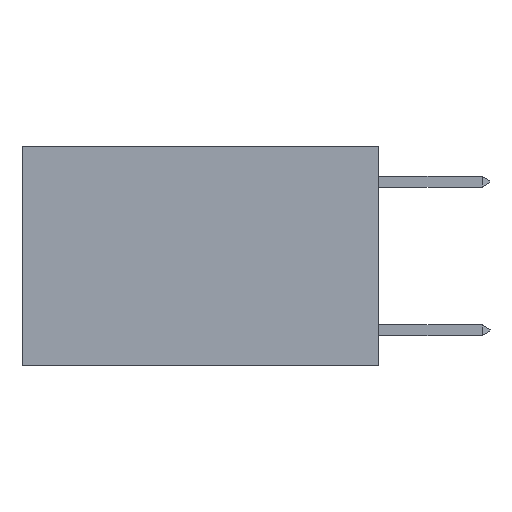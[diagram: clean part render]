
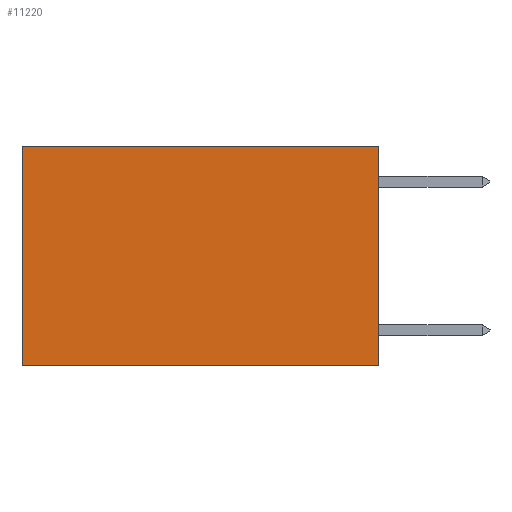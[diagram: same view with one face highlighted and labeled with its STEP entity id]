
A CAD part, left-side view. The second image highlights one B-rep face of the part: STEP entity #11220.
In plain terms, the highlighted planar face has unit normal (-1, 0, 0).
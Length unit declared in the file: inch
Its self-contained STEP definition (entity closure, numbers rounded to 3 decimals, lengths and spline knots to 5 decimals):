
#26 = VERTEX_POINT ( 'NONE', #25064 ) ;
#434 = CARTESIAN_POINT ( 'NONE',  ( 0.2625, 0.6, -0.37 ) ) ;
#883 = ORIENTED_EDGE ( 'NONE', *, *, #25227, .F. ) ;
#1131 = LINE ( 'NONE', #25044, #12066 ) ;
#1696 = VERTEX_POINT ( 'NONE', #16345 ) ;
#2349 = DIRECTION ( 'NONE',  ( 1., 0., 0. ) ) ;
#3793 = DIRECTION ( 'NONE',  ( 0., 1., 0. ) ) ;
#4288 = CARTESIAN_POINT ( 'NONE',  ( 0.2625, 0., 0. ) ) ;
#4978 = EDGE_CURVE ( 'NONE', #7265, #16873, #1131, .T. ) ;
#5120 = LINE ( 'NONE', #25198, #15955 ) ;
#5421 = EDGE_LOOP ( 'NONE', ( #12979, #883, #24620, #13647 ) ) ;
#6550 = DIRECTION ( 'NONE',  ( 0., 1., 0. ) ) ;
#7265 = VERTEX_POINT ( 'NONE', #19129 ) ;
#7379 = AXIS2_PLACEMENT_3D ( 'NONE', #25931, #2349, #17519 ) ;
#7971 = DIRECTION ( 'NONE',  ( 0., 0., -1. ) ) ;
#9309 = DIRECTION ( 'NONE',  ( 0., 0., -1. ) ) ;
#11220 = ADVANCED_FACE ( 'NONE', ( #26558 ), #23834, .F. ) ;
#12066 = VECTOR ( 'NONE', #7971, 39.37008 ) ;
#12979 = ORIENTED_EDGE ( 'NONE', *, *, #4978, .T. ) ;
#13647 = ORIENTED_EDGE ( 'NONE', *, *, #26670, .T. ) ;
#15797 = LINE ( 'NONE', #20091, #21474 ) ;
#15955 = VECTOR ( 'NONE', #3793, 39.37008 ) ;
#16345 = CARTESIAN_POINT ( 'NONE',  ( 0.2625, 0., -0.37 ) ) ;
#16873 = VERTEX_POINT ( 'NONE', #434 ) ;
#17519 = DIRECTION ( 'NONE',  ( 0., 0., -1. ) ) ;
#19129 = CARTESIAN_POINT ( 'NONE',  ( 0.2625, 0.6, 0. ) ) ;
#19543 = VECTOR ( 'NONE', #6550, 39.37008 ) ;
#20091 = CARTESIAN_POINT ( 'NONE',  ( 0.2625, 0., 0. ) ) ;
#21474 = VECTOR ( 'NONE', #9309, 39.37008 ) ;
#23834 = PLANE ( 'NONE',  #7379 ) ;
#24620 = ORIENTED_EDGE ( 'NONE', *, *, #27625, .F. ) ;
#25044 = CARTESIAN_POINT ( 'NONE',  ( 0.2625, 0.6, 0. ) ) ;
#25064 = CARTESIAN_POINT ( 'NONE',  ( 0.2625, 0., 0. ) ) ;
#25159 = LINE ( 'NONE', #4288, #19543 ) ;
#25198 = CARTESIAN_POINT ( 'NONE',  ( 0.2625, 0., -0.37 ) ) ;
#25227 = EDGE_CURVE ( 'NONE', #1696, #16873, #5120, .T. ) ;
#25931 = CARTESIAN_POINT ( 'NONE',  ( 0.2625, 0., 0. ) ) ;
#26558 = FACE_OUTER_BOUND ( 'NONE', #5421, .T. ) ;
#26670 = EDGE_CURVE ( 'NONE', #26, #7265, #25159, .T. ) ;
#27625 = EDGE_CURVE ( 'NONE', #26, #1696, #15797, .T. ) ;
